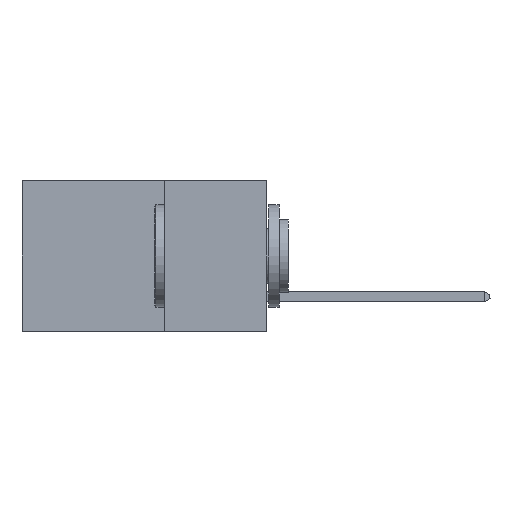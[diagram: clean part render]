
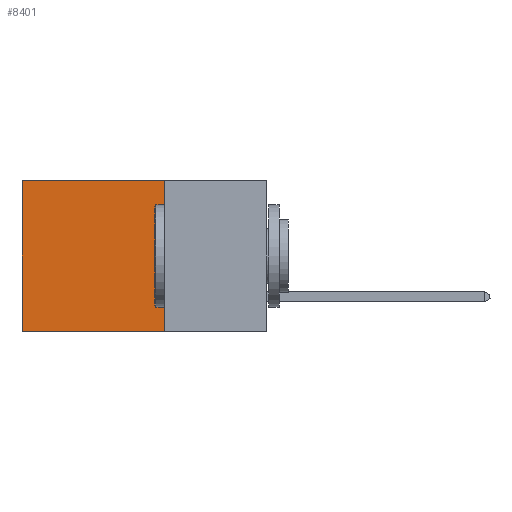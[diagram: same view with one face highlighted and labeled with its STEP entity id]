
A CAD part, left-side view. The second image highlights one B-rep face of the part: STEP entity #8401.
In plain terms, the highlighted planar face has unit normal (-1, 0, 0).
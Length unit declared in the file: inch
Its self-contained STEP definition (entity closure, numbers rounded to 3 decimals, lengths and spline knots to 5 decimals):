
#384 = VERTEX_POINT ( 'NONE', #4831 ) ;
#1739 = CARTESIAN_POINT ( 'NONE',  ( 0.2875, 0.6, 0. ) ) ;
#3769 = CARTESIAN_POINT ( 'NONE',  ( 0.2875, 0.25, 0. ) ) ;
#3839 = VERTEX_POINT ( 'NONE', #29232 ) ;
#3901 = DIRECTION ( 'NONE',  ( 0., 0., -1. ) ) ;
#4236 = EDGE_CURVE ( 'NONE', #16611, #384, #35097, .T. ) ;
#4831 = CARTESIAN_POINT ( 'NONE',  ( 0.2875, 0.6, -0.37 ) ) ;
#5497 = DIRECTION ( 'NONE',  ( 0., 0., -1. ) ) ;
#6615 = DIRECTION ( 'NONE',  ( 0., 1., 0. ) ) ;
#6966 = VECTOR ( 'NONE', #16639, 39.37008 ) ;
#8401 = ADVANCED_FACE ( 'NONE', ( #32238 ), #8479, .F. ) ;
#8479 = PLANE ( 'NONE',  #18443 ) ;
#10133 = CARTESIAN_POINT ( 'NONE',  ( 0.2875, 0.25, 0. ) ) ;
#10953 = VECTOR ( 'NONE', #3901, 39.37008 ) ;
#11084 = EDGE_CURVE ( 'NONE', #3839, #16611, #17649, .T. ) ;
#12877 = CARTESIAN_POINT ( 'NONE',  ( 0.2875, 0.25, -0.37 ) ) ;
#13052 = VERTEX_POINT ( 'NONE', #1739 ) ;
#14464 = CARTESIAN_POINT ( 'NONE',  ( 0.2875, 0.25, 0. ) ) ;
#16611 = VERTEX_POINT ( 'NONE', #17430 ) ;
#16639 = DIRECTION ( 'NONE',  ( 0., 1., 0. ) ) ;
#16762 = ORIENTED_EDGE ( 'NONE', *, *, #11084, .F. ) ;
#17049 = CARTESIAN_POINT ( 'NONE',  ( 0.2875, 0.6, 0. ) ) ;
#17430 = CARTESIAN_POINT ( 'NONE',  ( 0.2875, 0.25, -0.37 ) ) ;
#17649 = LINE ( 'NONE', #3769, #10953 ) ;
#18443 = AXIS2_PLACEMENT_3D ( 'NONE', #14464, #20574, #5497 ) ;
#19715 = VECTOR ( 'NONE', #6615, 39.37008 ) ;
#19888 = EDGE_CURVE ( 'NONE', #3839, #13052, #31329, .T. ) ;
#20536 = ORIENTED_EDGE ( 'NONE', *, *, #24370, .T. ) ;
#20574 = DIRECTION ( 'NONE',  ( 1., 0., 0. ) ) ;
#20934 = LINE ( 'NONE', #17049, #33417 ) ;
#22032 = ORIENTED_EDGE ( 'NONE', *, *, #4236, .F. ) ;
#22543 = ORIENTED_EDGE ( 'NONE', *, *, #19888, .T. ) ;
#24370 = EDGE_CURVE ( 'NONE', #13052, #384, #20934, .T. ) ;
#25587 = DIRECTION ( 'NONE',  ( 0., 0., -1. ) ) ;
#28942 = EDGE_LOOP ( 'NONE', ( #20536, #22032, #16762, #22543 ) ) ;
#29232 = CARTESIAN_POINT ( 'NONE',  ( 0.2875, 0.25, 0. ) ) ;
#31329 = LINE ( 'NONE', #10133, #6966 ) ;
#32238 = FACE_OUTER_BOUND ( 'NONE', #28942, .T. ) ;
#33417 = VECTOR ( 'NONE', #25587, 39.37008 ) ;
#35097 = LINE ( 'NONE', #12877, #19715 ) ;
